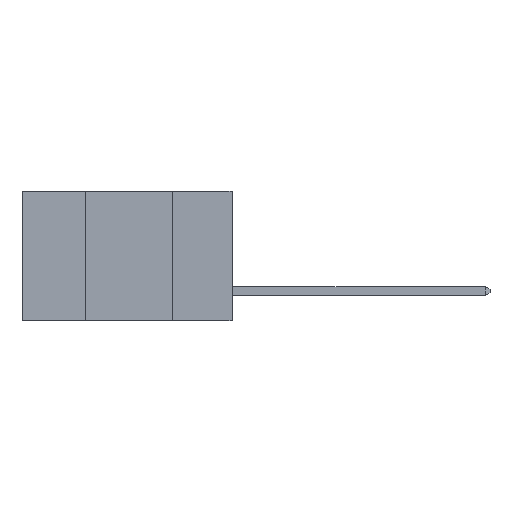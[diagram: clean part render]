
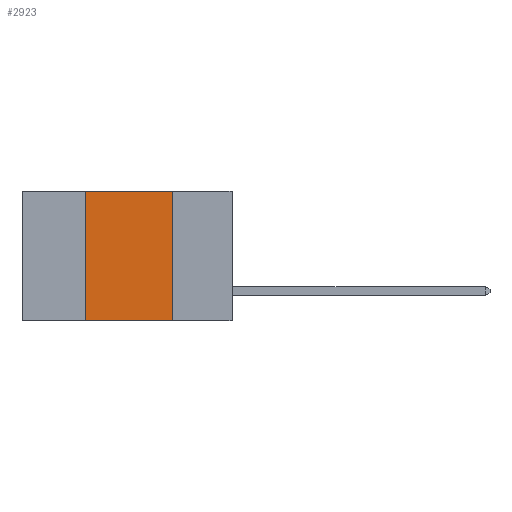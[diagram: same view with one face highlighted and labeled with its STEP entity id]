
A CAD part, left-side view. The second image highlights one B-rep face of the part: STEP entity #2923.
In plain terms, the highlighted planar face has unit normal (-1, 0, 0).
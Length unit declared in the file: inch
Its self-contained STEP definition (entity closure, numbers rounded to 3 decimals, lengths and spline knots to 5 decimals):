
#297 = VECTOR ( 'NONE', #6323, 39.37008 ) ;
#2923 = ADVANCED_FACE ( 'NONE', ( #20801 ), #16938, .F. ) ;
#3321 = CARTESIAN_POINT ( 'NONE',  ( 0., 0.17, -0.37 ) ) ;
#3645 = EDGE_CURVE ( 'NONE', #9932, #7991, #10203, .T. ) ;
#4319 = VERTEX_POINT ( 'NONE', #3321 ) ;
#4494 = DIRECTION ( 'NONE',  ( 0., -1., 0. ) ) ;
#5163 = CARTESIAN_POINT ( 'NONE',  ( 0., 0.42, 0. ) ) ;
#5314 = VECTOR ( 'NONE', #20232, 39.37008 ) ;
#5391 = CARTESIAN_POINT ( 'NONE',  ( 0., 0.42, -0.37 ) ) ;
#5413 = VECTOR ( 'NONE', #17829, 39.37008 ) ;
#5748 = LINE ( 'NONE', #11709, #297 ) ;
#6281 = EDGE_CURVE ( 'NONE', #11154, #4319, #14951, .T. ) ;
#6323 = DIRECTION ( 'NONE',  ( 0., -1., 0. ) ) ;
#7991 = VERTEX_POINT ( 'NONE', #5163 ) ;
#8370 = EDGE_CURVE ( 'NONE', #7991, #11154, #5748, .T. ) ;
#9830 = ORIENTED_EDGE ( 'NONE', *, *, #3645, .F. ) ;
#9932 = VERTEX_POINT ( 'NONE', #5391 ) ;
#10203 = LINE ( 'NONE', #19952, #5413 ) ;
#10799 = CARTESIAN_POINT ( 'NONE',  ( 0., 0.17, 0. ) ) ;
#11049 = CARTESIAN_POINT ( 'NONE',  ( 0., 0.17, 0. ) ) ;
#11110 = ORIENTED_EDGE ( 'NONE', *, *, #12743, .T. ) ;
#11154 = VERTEX_POINT ( 'NONE', #10799 ) ;
#11709 = CARTESIAN_POINT ( 'NONE',  ( 0., 0.6, 0. ) ) ;
#12166 = ORIENTED_EDGE ( 'NONE', *, *, #8370, .F. ) ;
#12585 = ORIENTED_EDGE ( 'NONE', *, *, #6281, .F. ) ;
#12743 = EDGE_CURVE ( 'NONE', #9932, #4319, #22450, .T. ) ;
#13772 = CARTESIAN_POINT ( 'NONE',  ( 0., 0.6, 0. ) ) ;
#14951 = LINE ( 'NONE', #11049, #5314 ) ;
#16495 = DIRECTION ( 'NONE',  ( 0., 0., -1. ) ) ;
#16635 = DIRECTION ( 'NONE',  ( 1., 0., 0. ) ) ;
#16938 = PLANE ( 'NONE',  #21985 ) ;
#17146 = CARTESIAN_POINT ( 'NONE',  ( 0., 0.6, -0.37 ) ) ;
#17829 = DIRECTION ( 'NONE',  ( 0., 0., 1. ) ) ;
#19249 = EDGE_LOOP ( 'NONE', ( #12585, #12166, #9830, #11110 ) ) ;
#19952 = CARTESIAN_POINT ( 'NONE',  ( 0., 0.42, 0. ) ) ;
#20232 = DIRECTION ( 'NONE',  ( 0., 0., -1. ) ) ;
#20801 = FACE_OUTER_BOUND ( 'NONE', #19249, .T. ) ;
#21985 = AXIS2_PLACEMENT_3D ( 'NONE', #13772, #16635, #16495 ) ;
#22450 = LINE ( 'NONE', #17146, #22990 ) ;
#22990 = VECTOR ( 'NONE', #4494, 39.37008 ) ;
